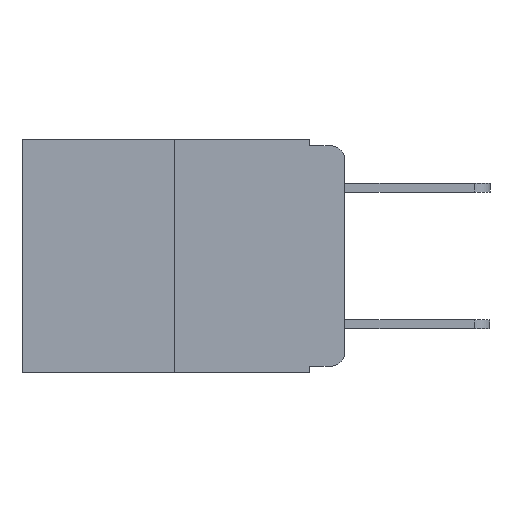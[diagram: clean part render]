
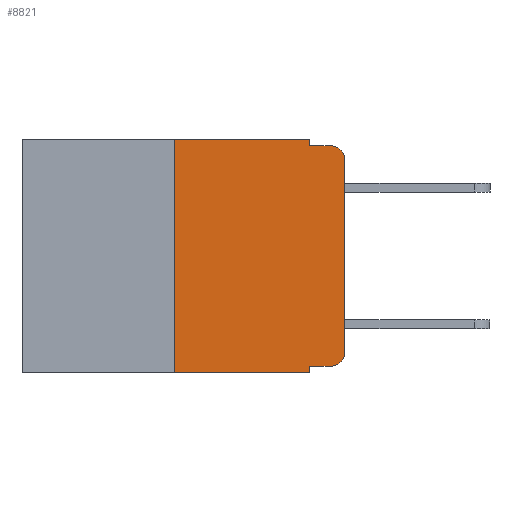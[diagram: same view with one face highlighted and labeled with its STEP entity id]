
A CAD part, left-side view. The second image highlights one B-rep face of the part: STEP entity #8821.
In plain terms, the highlighted planar face has unit normal (-1, 0, 0).
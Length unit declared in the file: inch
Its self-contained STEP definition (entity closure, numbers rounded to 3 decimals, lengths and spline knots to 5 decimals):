
#4 = DIRECTION ( 'NONE',  ( -1., 0., 0. ) ) ;
#10 = VERTEX_POINT ( 'NONE', #20741 ) ;
#552 = ORIENTED_EDGE ( 'NONE', *, *, #20963, .F. ) ;
#805 = CARTESIAN_POINT ( 'NONE',  ( 0., 0., -0.313 ) ) ;
#1580 = DIRECTION ( 'NONE',  ( 0., -1., 0. ) ) ;
#2258 = DIRECTION ( 'NONE',  ( 0., -1., 0. ) ) ;
#2304 = LINE ( 'NONE', #13247, #5493 ) ;
#2328 = LINE ( 'NONE', #2454, #6090 ) ;
#2386 = VERTEX_POINT ( 'NONE', #12555 ) ;
#2454 = CARTESIAN_POINT ( 'NONE',  ( 0., 0.25, 0. ) ) ;
#3265 = VECTOR ( 'NONE', #1580, 39.37008 ) ;
#3368 = CARTESIAN_POINT ( 'NONE',  ( 0., 0., -0.03 ) ) ;
#3821 = ORIENTED_EDGE ( 'NONE', *, *, #7895, .T. ) ;
#3932 = DIRECTION ( 'NONE',  ( 0., 0., -1. ) ) ;
#5306 = CARTESIAN_POINT ( 'NONE',  ( 0., 0.473, 0. ) ) ;
#5493 = VECTOR ( 'NONE', #2258, 39.37008 ) ;
#5499 = VECTOR ( 'NONE', #11452, 39.37008 ) ;
#5502 = VERTEX_POINT ( 'NONE', #805 ) ;
#6090 = VECTOR ( 'NONE', #18846, 39.37008 ) ;
#6712 = LINE ( 'NONE', #7739, #16934 ) ;
#6762 = EDGE_CURVE ( 'NONE', #15214, #16039, #12917, .T. ) ;
#7301 = VERTEX_POINT ( 'NONE', #18354 ) ;
#7385 = CARTESIAN_POINT ( 'NONE',  ( 0., 0., 0. ) ) ;
#7486 = AXIS2_PLACEMENT_3D ( 'NONE', #20918, #22699, #12008 ) ;
#7573 = CARTESIAN_POINT ( 'NONE',  ( 0., 0.051, 0. ) ) ;
#7739 = CARTESIAN_POINT ( 'NONE',  ( 0., 0.051, -0.333 ) ) ;
#7765 = CIRCLE ( 'NONE', #12593, 0.02 ) ;
#7895 = EDGE_CURVE ( 'NONE', #10, #5502, #13144, .T. ) ;
#8137 = LINE ( 'NONE', #5306, #3265 ) ;
#8274 = EDGE_LOOP ( 'NONE', ( #9034, #17252, #12537, #14244, #14051, #552, #15074, #15105, #21578, #3821 ) ) ;
#8306 = PLANE ( 'NONE',  #7486 ) ;
#8333 = LINE ( 'NONE', #19274, #22689 ) ;
#8489 = CARTESIAN_POINT ( 'NONE',  ( 0., 0.02, -0.01 ) ) ;
#8767 = DIRECTION ( 'NONE',  ( -1., 0., 0. ) ) ;
#8821 = ADVANCED_FACE ( 'NONE', ( #16764 ), #8306, .F. ) ;
#9034 = ORIENTED_EDGE ( 'NONE', *, *, #11097, .T. ) ;
#9090 = VERTEX_POINT ( 'NONE', #3368 ) ;
#9451 = VECTOR ( 'NONE', #3932, 39.37008 ) ;
#9978 = CARTESIAN_POINT ( 'NONE',  ( 0., 0.051, -0.343 ) ) ;
#10727 = VERTEX_POINT ( 'NONE', #15111 ) ;
#11016 = EDGE_CURVE ( 'NONE', #7301, #2386, #8137, .T. ) ;
#11090 = CARTESIAN_POINT ( 'NONE',  ( 0., 0.02, -0.313 ) ) ;
#11097 = EDGE_CURVE ( 'NONE', #5502, #9090, #11890, .T. ) ;
#11318 = VECTOR ( 'NONE', #12883, 39.37008 ) ;
#11434 = DIRECTION ( 'NONE',  ( 0., -1., 0. ) ) ;
#11452 = DIRECTION ( 'NONE',  ( 0., 0., -1. ) ) ;
#11484 = VERTEX_POINT ( 'NONE', #8489 ) ;
#11591 = VERTEX_POINT ( 'NONE', #19607 ) ;
#11890 = LINE ( 'NONE', #7385, #11318 ) ;
#12008 = DIRECTION ( 'NONE',  ( 0., 0., -1. ) ) ;
#12537 = ORIENTED_EDGE ( 'NONE', *, *, #21760, .F. ) ;
#12555 = CARTESIAN_POINT ( 'NONE',  ( 0., 0.051, 0. ) ) ;
#12593 = AXIS2_PLACEMENT_3D ( 'NONE', #19578, #8767, #21364 ) ;
#12880 = DIRECTION ( 'NONE',  ( 0., 0., -1. ) ) ;
#12883 = DIRECTION ( 'NONE',  ( 0., 0., 1. ) ) ;
#12917 = LINE ( 'NONE', #22159, #5499 ) ;
#13144 = CIRCLE ( 'NONE', #14777, 0.02 ) ;
#13247 = CARTESIAN_POINT ( 'NONE',  ( 0., 0.473, -0.343 ) ) ;
#13649 = EDGE_CURVE ( 'NONE', #2386, #11591, #19051, .T. ) ;
#14051 = ORIENTED_EDGE ( 'NONE', *, *, #11016, .F. ) ;
#14244 = ORIENTED_EDGE ( 'NONE', *, *, #13649, .F. ) ;
#14777 = AXIS2_PLACEMENT_3D ( 'NONE', #11090, #4, #12880 ) ;
#14851 = CARTESIAN_POINT ( 'NONE',  ( 0., 0.051, -0.333 ) ) ;
#15074 = ORIENTED_EDGE ( 'NONE', *, *, #22100, .T. ) ;
#15105 = ORIENTED_EDGE ( 'NONE', *, *, #6762, .F. ) ;
#15111 = CARTESIAN_POINT ( 'NONE',  ( 0., 0.25, -0.343 ) ) ;
#15214 = VERTEX_POINT ( 'NONE', #14851 ) ;
#16039 = VERTEX_POINT ( 'NONE', #9978 ) ;
#16764 = FACE_OUTER_BOUND ( 'NONE', #8274, .T. ) ;
#16934 = VECTOR ( 'NONE', #11434, 39.37008 ) ;
#17252 = ORIENTED_EDGE ( 'NONE', *, *, #22417, .T. ) ;
#18354 = CARTESIAN_POINT ( 'NONE',  ( 0., 0.25, 0. ) ) ;
#18846 = DIRECTION ( 'NONE',  ( 0., 0., 1. ) ) ;
#19051 = LINE ( 'NONE', #7573, #9451 ) ;
#19274 = CARTESIAN_POINT ( 'NONE',  ( 0., 0.051, -0.01 ) ) ;
#19578 = CARTESIAN_POINT ( 'NONE',  ( 0., 0.02, -0.03 ) ) ;
#19607 = CARTESIAN_POINT ( 'NONE',  ( 0., 0.051, -0.01 ) ) ;
#20129 = EDGE_CURVE ( 'NONE', #15214, #10, #6712, .T. ) ;
#20741 = CARTESIAN_POINT ( 'NONE',  ( 0., 0.02, -0.333 ) ) ;
#20918 = CARTESIAN_POINT ( 'NONE',  ( 0., 0.473, 0. ) ) ;
#20963 = EDGE_CURVE ( 'NONE', #10727, #7301, #2328, .T. ) ;
#21141 = DIRECTION ( 'NONE',  ( 0., -1., 0. ) ) ;
#21364 = DIRECTION ( 'NONE',  ( 0., 0., -1. ) ) ;
#21578 = ORIENTED_EDGE ( 'NONE', *, *, #20129, .T. ) ;
#21760 = EDGE_CURVE ( 'NONE', #11591, #11484, #8333, .T. ) ;
#22100 = EDGE_CURVE ( 'NONE', #10727, #16039, #2304, .T. ) ;
#22159 = CARTESIAN_POINT ( 'NONE',  ( 0., 0.051, 0. ) ) ;
#22417 = EDGE_CURVE ( 'NONE', #9090, #11484, #7765, .T. ) ;
#22689 = VECTOR ( 'NONE', #21141, 39.37008 ) ;
#22699 = DIRECTION ( 'NONE',  ( 1., 0., 0. ) ) ;
